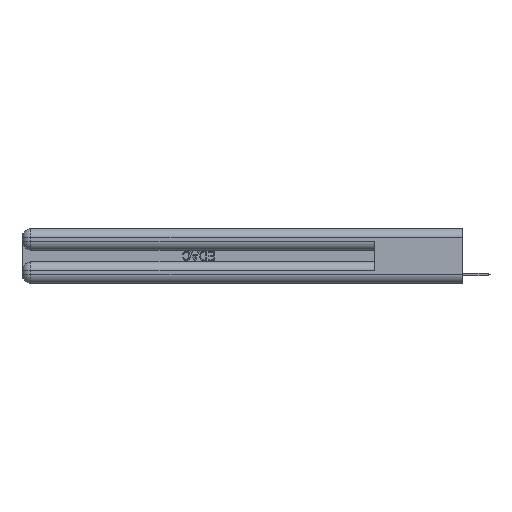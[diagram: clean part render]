
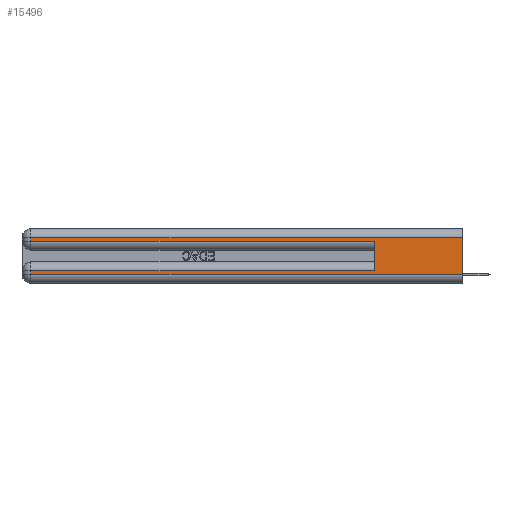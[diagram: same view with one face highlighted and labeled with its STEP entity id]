
A CAD part, left-side view. The second image highlights one B-rep face of the part: STEP entity #15496.
In plain terms, the highlighted planar face has unit normal (-1, 0, 0).
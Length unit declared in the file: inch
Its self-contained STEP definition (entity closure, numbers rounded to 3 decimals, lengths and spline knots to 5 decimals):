
#203 = EDGE_CURVE ( 'NONE', #25885, #24458, #6841, .T. ) ;
#541 = VECTOR ( 'NONE', #28203, 39.37008 ) ;
#690 = DIRECTION ( 'NONE',  ( 0., 0., -1. ) ) ;
#1149 = EDGE_CURVE ( 'NONE', #12438, #11093, #20939, .T. ) ;
#1193 = DIRECTION ( 'NONE',  ( 0., 1., 0. ) ) ;
#1314 = VECTOR ( 'NONE', #22913, 39.37008 ) ;
#1546 = EDGE_CURVE ( 'NONE', #18771, #2076, #28059, .T. ) ;
#2076 = VERTEX_POINT ( 'NONE', #17524 ) ;
#2220 = DIRECTION ( 'NONE',  ( 0., 0., -1. ) ) ;
#2989 = DIRECTION ( 'NONE',  ( 0., -1., 0. ) ) ;
#3227 = CARTESIAN_POINT ( 'NONE',  ( 0., 2.94, 0.31 ) ) ;
#3271 = EDGE_LOOP ( 'NONE', ( #24799, #22000, #21655, #8668, #10363, #18330, #11603, #8631 ) ) ;
#5836 = CARTESIAN_POINT ( 'NONE',  ( 0., 0., 0.37 ) ) ;
#6545 = VECTOR ( 'NONE', #1193, 39.37008 ) ;
#6576 = CARTESIAN_POINT ( 'NONE',  ( 0., 0., 0.37 ) ) ;
#6602 = CARTESIAN_POINT ( 'NONE',  ( 0., 0., 0.31 ) ) ;
#6717 = LINE ( 'NONE', #27804, #541 ) ;
#6841 = LINE ( 'NONE', #16537, #13020 ) ;
#7006 = DIRECTION ( 'NONE',  ( 0., 0., -1. ) ) ;
#7806 = VECTOR ( 'NONE', #2989, 39.37008 ) ;
#8631 = ORIENTED_EDGE ( 'NONE', *, *, #23087, .T. ) ;
#8668 = ORIENTED_EDGE ( 'NONE', *, *, #24133, .T. ) ;
#9456 = DIRECTION ( 'NONE',  ( 0., 0., 1. ) ) ;
#10174 = CARTESIAN_POINT ( 'NONE',  ( 0., 0.6, 0.285 ) ) ;
#10363 = ORIENTED_EDGE ( 'NONE', *, *, #1149, .F. ) ;
#10400 = CARTESIAN_POINT ( 'NONE',  ( 0., 0., 0.06 ) ) ;
#11093 = VERTEX_POINT ( 'NONE', #10174 ) ;
#11417 = PLANE ( 'NONE',  #26073 ) ;
#11488 = CARTESIAN_POINT ( 'NONE',  ( 0., 0.6, 0.145 ) ) ;
#11603 = ORIENTED_EDGE ( 'NONE', *, *, #1546, .T. ) ;
#12438 = VERTEX_POINT ( 'NONE', #19164 ) ;
#13020 = VECTOR ( 'NONE', #7006, 39.37008 ) ;
#13323 = EDGE_CURVE ( 'NONE', #12438, #18771, #27836, .T. ) ;
#13963 = LINE ( 'NONE', #14638, #7806 ) ;
#14222 = VECTOR ( 'NONE', #26538, 39.37008 ) ;
#14638 = CARTESIAN_POINT ( 'NONE',  ( 0., 0., 0.06 ) ) ;
#14879 = CARTESIAN_POINT ( 'NONE',  ( 0., 2.94, 0.37 ) ) ;
#15346 = LINE ( 'NONE', #5836, #14222 ) ;
#15452 = LINE ( 'NONE', #22512, #1314 ) ;
#15496 = ADVANCED_FACE ( 'NONE', ( #25198 ), #11417, .F. ) ;
#16537 = CARTESIAN_POINT ( 'NONE',  ( 0., 2.94, 0.37 ) ) ;
#17524 = CARTESIAN_POINT ( 'NONE',  ( 0., 2.94, 0.06 ) ) ;
#18317 = EDGE_CURVE ( 'NONE', #29197, #26034, #15346, .T. ) ;
#18330 = ORIENTED_EDGE ( 'NONE', *, *, #13323, .T. ) ;
#18771 = VERTEX_POINT ( 'NONE', #24484 ) ;
#19164 = CARTESIAN_POINT ( 'NONE',  ( 0., 0.6, 0.085 ) ) ;
#19693 = CARTESIAN_POINT ( 'NONE',  ( 0., 0., 0.085 ) ) ;
#20819 = CARTESIAN_POINT ( 'NONE',  ( 0., 2.94, 0.285 ) ) ;
#20939 = LINE ( 'NONE', #11488, #23092 ) ;
#21655 = ORIENTED_EDGE ( 'NONE', *, *, #203, .T. ) ;
#22000 = ORIENTED_EDGE ( 'NONE', *, *, #24022, .T. ) ;
#22512 = CARTESIAN_POINT ( 'NONE',  ( 0., 0., 0.31 ) ) ;
#22913 = DIRECTION ( 'NONE',  ( 0., 1., 0. ) ) ;
#23087 = EDGE_CURVE ( 'NONE', #2076, #26034, #13963, .T. ) ;
#23092 = VECTOR ( 'NONE', #9456, 39.37008 ) ;
#23765 = VECTOR ( 'NONE', #690, 39.37008 ) ;
#24022 = EDGE_CURVE ( 'NONE', #29197, #25885, #15452, .T. ) ;
#24133 = EDGE_CURVE ( 'NONE', #24458, #11093, #6717, .T. ) ;
#24458 = VERTEX_POINT ( 'NONE', #20819 ) ;
#24484 = CARTESIAN_POINT ( 'NONE',  ( 0., 2.94, 0.085 ) ) ;
#24799 = ORIENTED_EDGE ( 'NONE', *, *, #18317, .F. ) ;
#25198 = FACE_OUTER_BOUND ( 'NONE', #3271, .T. ) ;
#25885 = VERTEX_POINT ( 'NONE', #3227 ) ;
#26034 = VERTEX_POINT ( 'NONE', #10400 ) ;
#26073 = AXIS2_PLACEMENT_3D ( 'NONE', #6576, #29845, #2220 ) ;
#26538 = DIRECTION ( 'NONE',  ( 0., 0., -1. ) ) ;
#27804 = CARTESIAN_POINT ( 'NONE',  ( 0., 0., 0.285 ) ) ;
#27836 = LINE ( 'NONE', #19693, #6545 ) ;
#28059 = LINE ( 'NONE', #14879, #23765 ) ;
#28203 = DIRECTION ( 'NONE',  ( 0., -1., 0. ) ) ;
#29197 = VERTEX_POINT ( 'NONE', #6602 ) ;
#29845 = DIRECTION ( 'NONE',  ( 1., 0., 0. ) ) ;
